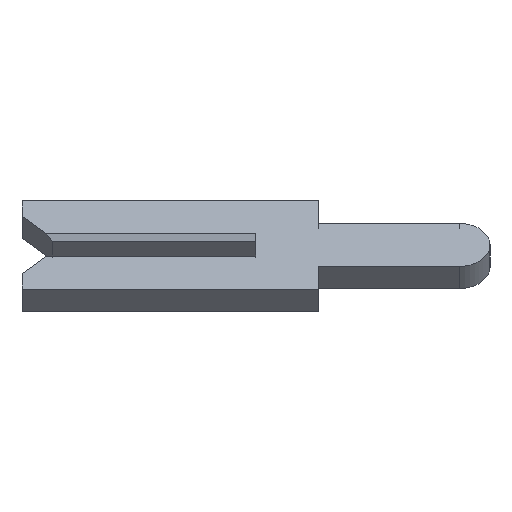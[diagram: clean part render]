
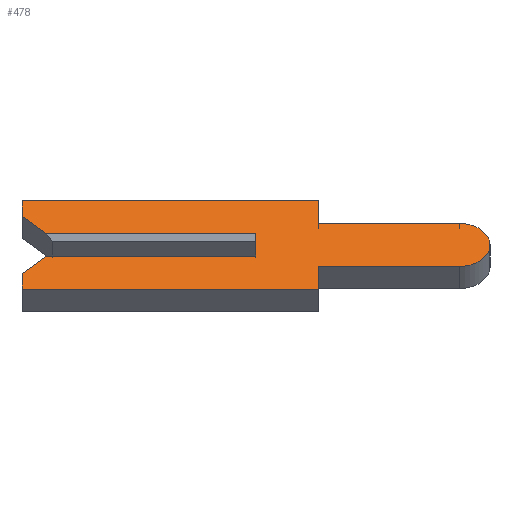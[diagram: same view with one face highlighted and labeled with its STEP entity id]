
A CAD part, left-side view. The second image highlights one B-rep face of the part: STEP entity #478.
In plain terms, the highlighted face is planar.
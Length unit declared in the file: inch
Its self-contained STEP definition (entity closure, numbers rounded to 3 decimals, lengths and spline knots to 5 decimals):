
#1 = ORIENTED_EDGE ( 'NONE', *, *, #212, .F. ) ;
#17 = VERTEX_POINT ( 'NONE', #770 ) ;
#28 = VECTOR ( 'NONE', #793, 39.37008 ) ;
#35 = LINE ( 'NONE', #1010, #479 ) ;
#45 = DIRECTION ( 'NONE',  ( 0., 0., -1. ) ) ;
#53 = DIRECTION ( 'NONE',  ( 1., 0., 0. ) ) ;
#68 = CARTESIAN_POINT ( 'NONE',  ( -0.01, -0.04, -0.0195 ) ) ;
#75 = LINE ( 'NONE', #831, #789 ) ;
#78 = CARTESIAN_POINT ( 'NONE',  ( -0.01, 0.1305, -0.0065 ) ) ;
#87 = CARTESIAN_POINT ( 'NONE',  ( -0.01, -0.04, -0.04 ) ) ;
#97 = CARTESIAN_POINT ( 'NONE',  ( -0.01, 0.15, 0.04 ) ) ;
#101 = CARTESIAN_POINT ( 'NONE',  ( -0.01, -0.04, 0.0195 ) ) ;
#105 = DIRECTION ( 'NONE',  ( 0., -1., 0. ) ) ;
#115 = DIRECTION ( 'NONE',  ( 0., 0., 1. ) ) ;
#126 = CARTESIAN_POINT ( 'NONE',  ( -0.01, 0.15, 0.026 ) ) ;
#128 = VERTEX_POINT ( 'NONE', #591 ) ;
#147 = LINE ( 'NONE', #265, #321 ) ;
#148 = CARTESIAN_POINT ( 'NONE',  ( -0.01, 0.15, -0.026 ) ) ;
#150 = VECTOR ( 'NONE', #115, 39.37008 ) ;
#163 = VERTEX_POINT ( 'NONE', #262 ) ;
#188 = CARTESIAN_POINT ( 'NONE',  ( -0.01, 0., -0.01 ) ) ;
#189 = CARTESIAN_POINT ( 'NONE',  ( -0.01, -0.04, -0.04 ) ) ;
#191 = VECTOR ( 'NONE', #105, 39.37008 ) ;
#211 = VECTOR ( 'NONE', #643, 39.37008 ) ;
#212 = EDGE_CURVE ( 'NONE', #871, #802, #1059, .T. ) ;
#215 = VERTEX_POINT ( 'NONE', #430 ) ;
#216 = ORIENTED_EDGE ( 'NONE', *, *, #544, .F. ) ;
#223 = ORIENTED_EDGE ( 'NONE', *, *, #865, .F. ) ;
#231 = LINE ( 'NONE', #126, #150 ) ;
#232 = EDGE_CURVE ( 'NONE', #163, #871, #893, .T. ) ;
#240 = VERTEX_POINT ( 'NONE', #97 ) ;
#241 = VERTEX_POINT ( 'NONE', #606 ) ;
#242 = DIRECTION ( 'NONE',  ( 0., 1., 0. ) ) ;
#262 = CARTESIAN_POINT ( 'NONE',  ( -0.01, -0.1305, 0.0195 ) ) ;
#265 = CARTESIAN_POINT ( 'NONE',  ( -0.01, -0.1305, -0.01 ) ) ;
#266 = CARTESIAN_POINT ( 'NONE',  ( -0.01, 0.15, 0.04 ) ) ;
#271 = EDGE_CURVE ( 'NONE', #241, #163, #807, .T. ) ;
#277 = FACE_OUTER_BOUND ( 'NONE', #398, .T. ) ;
#280 = EDGE_CURVE ( 'NONE', #802, #818, #1083, .T. ) ;
#287 = LINE ( 'NONE', #78, #1086 ) ;
#290 = VERTEX_POINT ( 'NONE', #349 ) ;
#303 = ORIENTED_EDGE ( 'NONE', *, *, #343, .F. ) ;
#309 = EDGE_CURVE ( 'NONE', #240, #128, #455, .T. ) ;
#321 = VECTOR ( 'NONE', #370, 39.37008 ) ;
#343 = EDGE_CURVE ( 'NONE', #290, #1043, #147, .T. ) ;
#344 = DIRECTION ( 'NONE',  ( 0., 1., 0. ) ) ;
#349 = CARTESIAN_POINT ( 'NONE',  ( -0.01, 0.134, -0.01 ) ) ;
#370 = DIRECTION ( 'NONE',  ( 0., -1., 0. ) ) ;
#398 = EDGE_LOOP ( 'NONE', ( #776, #498, #303, #991, #971, #223, #884, #1, #485, #652, #700, #738, #216, #520 ) ) ;
#399 = EDGE_CURVE ( 'NONE', #215, #1038, #725, .T. ) ;
#408 = VECTOR ( 'NONE', #717, 39.37008 ) ;
#422 = LINE ( 'NONE', #148, #983 ) ;
#430 = CARTESIAN_POINT ( 'NONE',  ( -0.01, 0.134, 0.01 ) ) ;
#439 = DIRECTION ( 'NONE',  ( 0., -1., 0. ) ) ;
#453 = AXIS2_PLACEMENT_3D ( 'NONE', #964, #712, #967 ) ;
#455 = LINE ( 'NONE', #266, #191 ) ;
#476 = CARTESIAN_POINT ( 'NONE',  ( -0.01, -0.04, 0.04 ) ) ;
#478 = ADVANCED_FACE ( 'NONE', ( #277 ), #891, .F. ) ;
#479 = VECTOR ( 'NONE', #242, 39.37008 ) ;
#485 = ORIENTED_EDGE ( 'NONE', *, *, #232, .F. ) ;
#498 = ORIENTED_EDGE ( 'NONE', *, *, #592, .F. ) ;
#508 = CARTESIAN_POINT ( 'NONE',  ( -0.01, -0.04, -0.0195 ) ) ;
#520 = ORIENTED_EDGE ( 'NONE', *, *, #935, .F. ) ;
#544 = EDGE_CURVE ( 'NONE', #17, #240, #231, .T. ) ;
#561 = AXIS2_PLACEMENT_3D ( 'NONE', #1068, #53, #45 ) ;
#574 = VECTOR ( 'NONE', #1019, 39.37008 ) ;
#591 = CARTESIAN_POINT ( 'NONE',  ( -0.01, -0.04, 0.04 ) ) ;
#592 = EDGE_CURVE ( 'NONE', #1043, #1038, #75, .T. ) ;
#593 = CARTESIAN_POINT ( 'NONE',  ( -0.01, -0.1305, -0.0195 ) ) ;
#606 = CARTESIAN_POINT ( 'NONE',  ( -0.01, -0.04, 0.0195 ) ) ;
#637 = LINE ( 'NONE', #476, #211 ) ;
#638 = VECTOR ( 'NONE', #344, 39.37008 ) ;
#643 = DIRECTION ( 'NONE',  ( 0., 0., -1. ) ) ;
#645 = EDGE_CURVE ( 'NONE', #1084, #881, #422, .T. ) ;
#652 = ORIENTED_EDGE ( 'NONE', *, *, #271, .F. ) ;
#653 = VECTOR ( 'NONE', #439, 39.37008 ) ;
#656 = DIRECTION ( 'NONE',  ( 0., 0., 1. ) ) ;
#700 = ORIENTED_EDGE ( 'NONE', *, *, #742, .F. ) ;
#712 = DIRECTION ( 'NONE',  ( 1., 0., 0. ) ) ;
#717 = DIRECTION ( 'NONE',  ( 0., -1., 0. ) ) ;
#725 = LINE ( 'NONE', #883, #408 ) ;
#738 = ORIENTED_EDGE ( 'NONE', *, *, #309, .F. ) ;
#742 = EDGE_CURVE ( 'NONE', #128, #241, #637, .T. ) ;
#758 = CARTESIAN_POINT ( 'NONE',  ( -0.01, 0.15, -0.026 ) ) ;
#770 = CARTESIAN_POINT ( 'NONE',  ( -0.01, 0.15, 0.026 ) ) ;
#776 = ORIENTED_EDGE ( 'NONE', *, *, #399, .T. ) ;
#789 = VECTOR ( 'NONE', #656, 39.37008 ) ;
#793 = DIRECTION ( 'NONE',  ( 0., 0., -1. ) ) ;
#797 = LINE ( 'NONE', #1015, #574 ) ;
#802 = VERTEX_POINT ( 'NONE', #68 ) ;
#807 = LINE ( 'NONE', #101, #653 ) ;
#818 = VERTEX_POINT ( 'NONE', #87 ) ;
#824 = DIRECTION ( 'NONE',  ( 0., 0., 1. ) ) ;
#831 = CARTESIAN_POINT ( 'NONE',  ( -0.01, 0., 0.0065 ) ) ;
#849 = DIRECTION ( 'NONE',  ( 0., -0.707, 0.707 ) ) ;
#865 = EDGE_CURVE ( 'NONE', #818, #1084, #35, .T. ) ;
#871 = VERTEX_POINT ( 'NONE', #593 ) ;
#881 = VERTEX_POINT ( 'NONE', #758 ) ;
#883 = CARTESIAN_POINT ( 'NONE',  ( -0.01, 0.15, 0.01 ) ) ;
#884 = ORIENTED_EDGE ( 'NONE', *, *, #280, .F. ) ;
#891 = PLANE ( 'NONE',  #561 ) ;
#893 = CIRCLE ( 'NONE', #453, 0.0195 ) ;
#935 = EDGE_CURVE ( 'NONE', #215, #17, #797, .T. ) ;
#945 = EDGE_CURVE ( 'NONE', #881, #290, #287, .T. ) ;
#960 = CARTESIAN_POINT ( 'NONE',  ( -0.01, 0., 0.01 ) ) ;
#964 = CARTESIAN_POINT ( 'NONE',  ( -0.01, -0.1305, 0. ) ) ;
#967 = DIRECTION ( 'NONE',  ( 0., 0., -1. ) ) ;
#971 = ORIENTED_EDGE ( 'NONE', *, *, #645, .F. ) ;
#983 = VECTOR ( 'NONE', #824, 39.37008 ) ;
#991 = ORIENTED_EDGE ( 'NONE', *, *, #945, .F. ) ;
#1010 = CARTESIAN_POINT ( 'NONE',  ( -0.01, 0.15, -0.04 ) ) ;
#1015 = CARTESIAN_POINT ( 'NONE',  ( -0.01, 0.1305, 0.0065 ) ) ;
#1019 = DIRECTION ( 'NONE',  ( 0., 0.707, 0.707 ) ) ;
#1031 = CARTESIAN_POINT ( 'NONE',  ( -0.01, 0.15, -0.04 ) ) ;
#1038 = VERTEX_POINT ( 'NONE', #960 ) ;
#1043 = VERTEX_POINT ( 'NONE', #188 ) ;
#1059 = LINE ( 'NONE', #508, #638 ) ;
#1068 = CARTESIAN_POINT ( 'NONE',  ( -0.01, -0.1305, 0. ) ) ;
#1083 = LINE ( 'NONE', #189, #28 ) ;
#1084 = VERTEX_POINT ( 'NONE', #1031 ) ;
#1086 = VECTOR ( 'NONE', #849, 39.37008 ) ;
